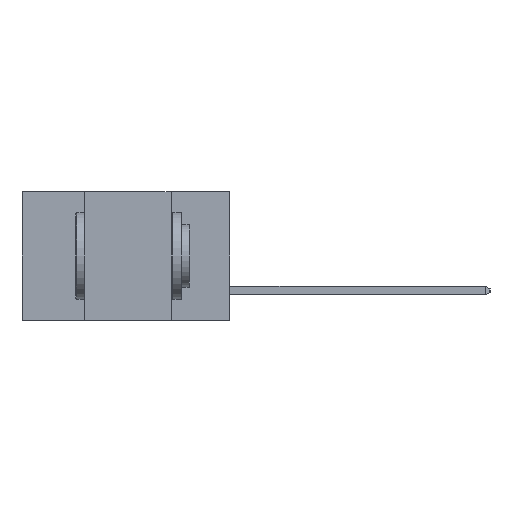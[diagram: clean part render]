
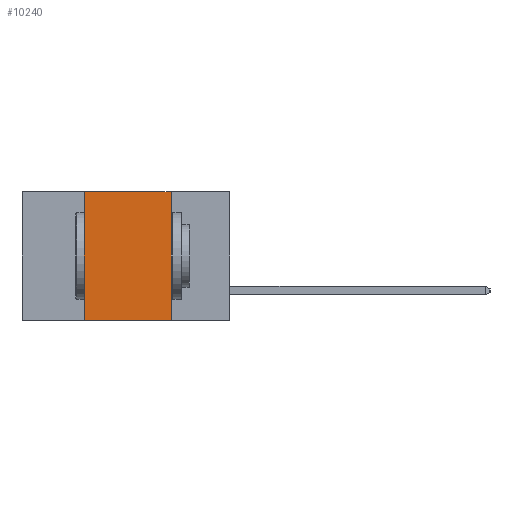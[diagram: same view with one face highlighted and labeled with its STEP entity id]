
A CAD part, left-side view. The second image highlights one B-rep face of the part: STEP entity #10240.
In plain terms, the highlighted planar face has unit normal (-1, 0, 0).
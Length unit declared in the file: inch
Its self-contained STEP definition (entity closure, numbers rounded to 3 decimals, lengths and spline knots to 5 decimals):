
#196 = VERTEX_POINT ( 'NONE', #5342 ) ;
#267 = LINE ( 'NONE', #6141, #7888 ) ;
#710 = EDGE_CURVE ( 'NONE', #15970, #1831, #5217, .T. ) ;
#799 = VERTEX_POINT ( 'NONE', #17376 ) ;
#1515 = PLANE ( 'NONE',  #11073 ) ;
#1831 = VERTEX_POINT ( 'NONE', #18137 ) ;
#1993 = LINE ( 'NONE', #4124, #17547 ) ;
#4124 = CARTESIAN_POINT ( 'NONE',  ( 0., 0.6, -0.37 ) ) ;
#4585 = CARTESIAN_POINT ( 'NONE',  ( 0., 0.6, 0. ) ) ;
#5217 = LINE ( 'NONE', #6180, #12695 ) ;
#5342 = CARTESIAN_POINT ( 'NONE',  ( 0., 0.17, -0.37 ) ) ;
#5434 = CARTESIAN_POINT ( 'NONE',  ( 0., 0.42, 0. ) ) ;
#5841 = FACE_OUTER_BOUND ( 'NONE', #14632, .T. ) ;
#6120 = DIRECTION ( 'NONE',  ( 0., 0., -1. ) ) ;
#6141 = CARTESIAN_POINT ( 'NONE',  ( 0., 0.17, 0. ) ) ;
#6180 = CARTESIAN_POINT ( 'NONE',  ( 0., 0.6, 0. ) ) ;
#7888 = VECTOR ( 'NONE', #12121, 39.37008 ) ;
#8674 = ORIENTED_EDGE ( 'NONE', *, *, #17768, .F. ) ;
#8795 = DIRECTION ( 'NONE',  ( 0., -1., 0. ) ) ;
#10240 = ADVANCED_FACE ( 'NONE', ( #5841 ), #1515, .F. ) ;
#10251 = ORIENTED_EDGE ( 'NONE', *, *, #710, .F. ) ;
#10320 = ORIENTED_EDGE ( 'NONE', *, *, #12699, .T. ) ;
#10917 = VECTOR ( 'NONE', #16009, 39.37008 ) ;
#11073 = AXIS2_PLACEMENT_3D ( 'NONE', #4585, #15177, #6120 ) ;
#12121 = DIRECTION ( 'NONE',  ( 0., 0., -1. ) ) ;
#12695 = VECTOR ( 'NONE', #8795, 39.37008 ) ;
#12699 = EDGE_CURVE ( 'NONE', #799, #196, #1993, .T. ) ;
#12906 = CARTESIAN_POINT ( 'NONE',  ( 0., 0.42, 0. ) ) ;
#14632 = EDGE_LOOP ( 'NONE', ( #8674, #10251, #16988, #10320 ) ) ;
#15025 = LINE ( 'NONE', #12906, #10917 ) ;
#15177 = DIRECTION ( 'NONE',  ( 1., 0., 0. ) ) ;
#15970 = VERTEX_POINT ( 'NONE', #5434 ) ;
#16009 = DIRECTION ( 'NONE',  ( 0., 0., 1. ) ) ;
#16222 = DIRECTION ( 'NONE',  ( 0., -1., 0. ) ) ;
#16791 = EDGE_CURVE ( 'NONE', #799, #15970, #15025, .T. ) ;
#16988 = ORIENTED_EDGE ( 'NONE', *, *, #16791, .F. ) ;
#17376 = CARTESIAN_POINT ( 'NONE',  ( 0., 0.42, -0.37 ) ) ;
#17547 = VECTOR ( 'NONE', #16222, 39.37008 ) ;
#17768 = EDGE_CURVE ( 'NONE', #1831, #196, #267, .T. ) ;
#18137 = CARTESIAN_POINT ( 'NONE',  ( 0., 0.17, 0. ) ) ;
